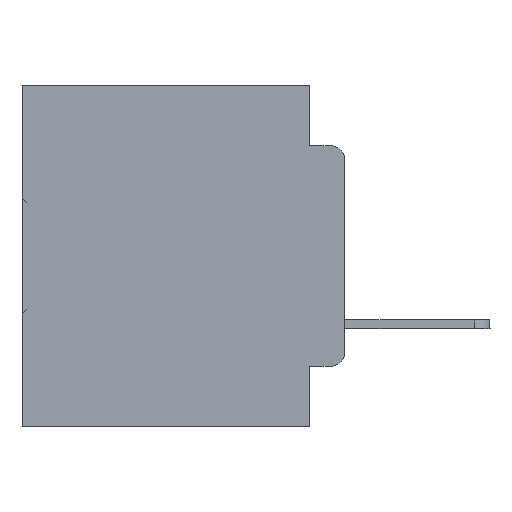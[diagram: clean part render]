
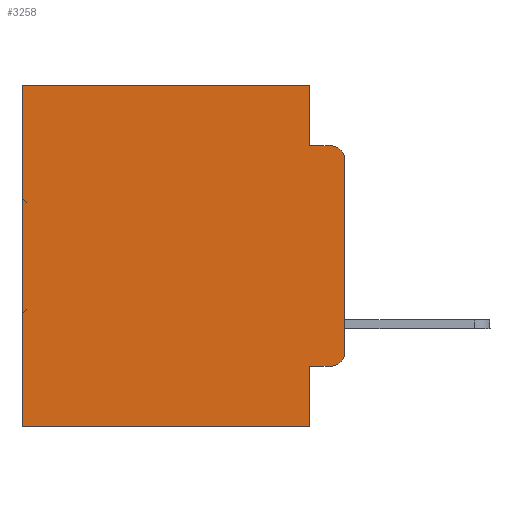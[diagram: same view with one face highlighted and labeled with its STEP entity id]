
A CAD part, left-side view. The second image highlights one B-rep face of the part: STEP entity #3258.
In plain terms, the highlighted planar face has unit normal (-1, 0, 0).
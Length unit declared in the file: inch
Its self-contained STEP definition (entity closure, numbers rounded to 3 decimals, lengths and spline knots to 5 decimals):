
#139 = VERTEX_POINT ( 'NONE', #14224 ) ;
#349 = CARTESIAN_POINT ( 'NONE',  ( 0.298, 0.051, -0.4115 ) ) ;
#372 = CIRCLE ( 'NONE', #15701, 0.02 ) ;
#483 = VECTOR ( 'NONE', #11733, 39.37008 ) ;
#748 = VECTOR ( 'NONE', #32194, 39.37008 ) ;
#2908 = VERTEX_POINT ( 'NONE', #25162 ) ;
#3200 = VERTEX_POINT ( 'NONE', #7881 ) ;
#3258 = ADVANCED_FACE ( 'NONE', ( #33380 ), #5158, .F. ) ;
#3577 = DIRECTION ( 'NONE',  ( 0., 0., -1. ) ) ;
#4270 = DIRECTION ( 'NONE',  ( 0., 0., -1. ) ) ;
#4465 = VECTOR ( 'NONE', #4270, 39.37008 ) ;
#5158 = PLANE ( 'NONE',  #31786 ) ;
#5193 = VERTEX_POINT ( 'NONE', #17818 ) ;
#6027 = CARTESIAN_POINT ( 'NONE',  ( 0.298, 0., -0.5 ) ) ;
#6080 = VECTOR ( 'NONE', #24656, 39.37008 ) ;
#6577 = LINE ( 'NONE', #9800, #4465 ) ;
#6647 = DIRECTION ( 'NONE',  ( 0., 0., -1. ) ) ;
#7044 = CARTESIAN_POINT ( 'NONE',  ( 0.298, 0.051, -0.5 ) ) ;
#7385 = EDGE_CURVE ( 'NONE', #31010, #2908, #9919, .T. ) ;
#7881 = CARTESIAN_POINT ( 'NONE',  ( 0.298, 0., -0.1085 ) ) ;
#8590 = VERTEX_POINT ( 'NONE', #15173 ) ;
#9258 = CARTESIAN_POINT ( 'NONE',  ( 0.298, 0., 0. ) ) ;
#9520 = VECTOR ( 'NONE', #34312, 39.37008 ) ;
#9800 = CARTESIAN_POINT ( 'NONE',  ( 0.298, 0.051, 0. ) ) ;
#9813 = CARTESIAN_POINT ( 'NONE',  ( 0.298, 0.02, -0.4115 ) ) ;
#9918 = ORIENTED_EDGE ( 'NONE', *, *, #16797, .F. ) ;
#9919 = LINE ( 'NONE', #25001, #20842 ) ;
#10218 = CARTESIAN_POINT ( 'NONE',  ( 0.298, 0.051, -0.0885 ) ) ;
#10485 = EDGE_CURVE ( 'NONE', #3200, #25573, #28200, .T. ) ;
#10674 = ORIENTED_EDGE ( 'NONE', *, *, #19770, .T. ) ;
#11340 = ORIENTED_EDGE ( 'NONE', *, *, #20017, .F. ) ;
#11733 = DIRECTION ( 'NONE',  ( 0., 1., 0. ) ) ;
#12054 = VERTEX_POINT ( 'NONE', #14219 ) ;
#12189 = VERTEX_POINT ( 'NONE', #9813 ) ;
#13041 = AXIS2_PLACEMENT_3D ( 'NONE', #33230, #22872, #6647 ) ;
#13115 = VERTEX_POINT ( 'NONE', #7044 ) ;
#13346 = CARTESIAN_POINT ( 'NONE',  ( 0.298, 0., 0. ) ) ;
#14219 = CARTESIAN_POINT ( 'NONE',  ( 0.298, 0.051, -0.0885 ) ) ;
#14224 = CARTESIAN_POINT ( 'NONE',  ( 0.298, 0.02, -0.0885 ) ) ;
#14520 = DIRECTION ( 'NONE',  ( 0., 0., -1. ) ) ;
#15152 = CARTESIAN_POINT ( 'NONE',  ( 0.298, 0.051, 0. ) ) ;
#15173 = CARTESIAN_POINT ( 'NONE',  ( 0.298, 0.051, 0. ) ) ;
#15242 = ORIENTED_EDGE ( 'NONE', *, *, #10485, .F. ) ;
#15701 = AXIS2_PLACEMENT_3D ( 'NONE', #28988, #18267, #28643 ) ;
#16316 = ORIENTED_EDGE ( 'NONE', *, *, #23304, .T. ) ;
#16797 = EDGE_CURVE ( 'NONE', #8590, #12054, #28508, .T. ) ;
#17818 = CARTESIAN_POINT ( 'NONE',  ( 0.298, 0.051, -0.4115 ) ) ;
#18267 = DIRECTION ( 'NONE',  ( -1., 0., 0. ) ) ;
#18281 = EDGE_CURVE ( 'NONE', #8590, #31010, #24149, .T. ) ;
#19109 = CARTESIAN_POINT ( 'NONE',  ( 0.298, 0.473, 0. ) ) ;
#19770 = EDGE_CURVE ( 'NONE', #3200, #139, #372, .T. ) ;
#20017 = EDGE_CURVE ( 'NONE', #13115, #2908, #26557, .T. ) ;
#20633 = LINE ( 'NONE', #10218, #29520 ) ;
#20842 = VECTOR ( 'NONE', #3577, 39.37008 ) ;
#21378 = ORIENTED_EDGE ( 'NONE', *, *, #30348, .T. ) ;
#22494 = CARTESIAN_POINT ( 'NONE',  ( 0.298, 0., 0. ) ) ;
#22859 = EDGE_CURVE ( 'NONE', #5193, #13115, #6577, .T. ) ;
#22872 = DIRECTION ( 'NONE',  ( -1., 0., 0. ) ) ;
#23304 = EDGE_CURVE ( 'NONE', #12189, #25573, #23410, .T. ) ;
#23410 = CIRCLE ( 'NONE', #13041, 0.02 ) ;
#23856 = EDGE_LOOP ( 'NONE', ( #15242, #10674, #29351, #9918, #33038, #23962, #11340, #25159, #21378, #16316 ) ) ;
#23962 = ORIENTED_EDGE ( 'NONE', *, *, #7385, .T. ) ;
#24149 = LINE ( 'NONE', #9258, #483 ) ;
#24656 = DIRECTION ( 'NONE',  ( 0., -1., 0. ) ) ;
#24855 = DIRECTION ( 'NONE',  ( 0., 1., 0. ) ) ;
#25001 = CARTESIAN_POINT ( 'NONE',  ( 0.298, 0.473, 0. ) ) ;
#25159 = ORIENTED_EDGE ( 'NONE', *, *, #22859, .F. ) ;
#25162 = CARTESIAN_POINT ( 'NONE',  ( 0.298, 0.473, -0.5 ) ) ;
#25223 = DIRECTION ( 'NONE',  ( 1., 0., 0. ) ) ;
#25573 = VERTEX_POINT ( 'NONE', #32577 ) ;
#25909 = LINE ( 'NONE', #349, #6080 ) ;
#26557 = LINE ( 'NONE', #6027, #32016 ) ;
#26908 = EDGE_CURVE ( 'NONE', #12054, #139, #20633, .T. ) ;
#28200 = LINE ( 'NONE', #13346, #748 ) ;
#28508 = LINE ( 'NONE', #15152, #9520 ) ;
#28643 = DIRECTION ( 'NONE',  ( 0., 0., -1. ) ) ;
#28988 = CARTESIAN_POINT ( 'NONE',  ( 0.298, 0.02, -0.1085 ) ) ;
#29351 = ORIENTED_EDGE ( 'NONE', *, *, #26908, .F. ) ;
#29520 = VECTOR ( 'NONE', #31542, 39.37008 ) ;
#30348 = EDGE_CURVE ( 'NONE', #5193, #12189, #25909, .T. ) ;
#31010 = VERTEX_POINT ( 'NONE', #19109 ) ;
#31542 = DIRECTION ( 'NONE',  ( 0., -1., 0. ) ) ;
#31786 = AXIS2_PLACEMENT_3D ( 'NONE', #22494, #25223, #14520 ) ;
#32016 = VECTOR ( 'NONE', #24855, 39.37008 ) ;
#32194 = DIRECTION ( 'NONE',  ( 0., 0., -1. ) ) ;
#32577 = CARTESIAN_POINT ( 'NONE',  ( 0.298, 0., -0.3915 ) ) ;
#33038 = ORIENTED_EDGE ( 'NONE', *, *, #18281, .T. ) ;
#33230 = CARTESIAN_POINT ( 'NONE',  ( 0.298, 0.02, -0.3915 ) ) ;
#33380 = FACE_OUTER_BOUND ( 'NONE', #23856, .T. ) ;
#34312 = DIRECTION ( 'NONE',  ( 0., 0., -1. ) ) ;
